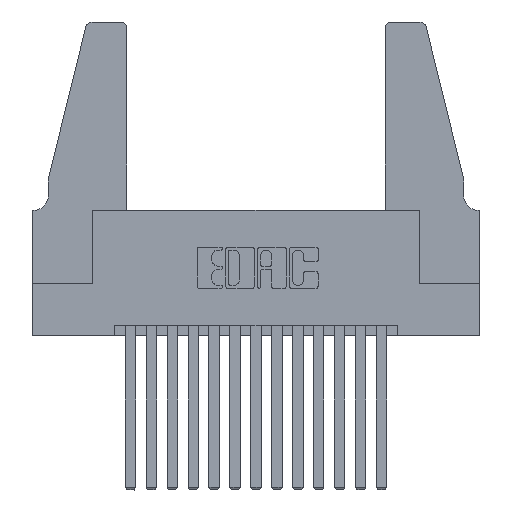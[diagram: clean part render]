
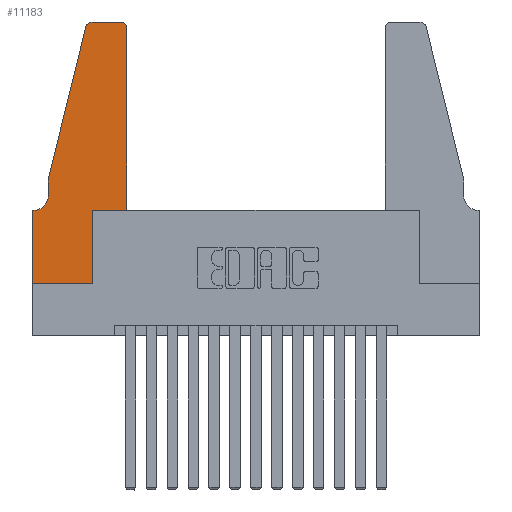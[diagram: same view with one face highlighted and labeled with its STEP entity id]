
A CAD part, top view. The second image highlights one B-rep face of the part: STEP entity #11183.
In plain terms, the highlighted planar face has unit normal (0, 0, 1).
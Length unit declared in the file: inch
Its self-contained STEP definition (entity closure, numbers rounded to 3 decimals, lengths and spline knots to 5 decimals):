
#358 = VERTEX_POINT ( 'NONE', #2515 ) ;
#392 = CARTESIAN_POINT ( 'NONE',  ( 0.0755, 0.42, 0.37 ) ) ;
#960 = VECTOR ( 'NONE', #9195, 39.37008 ) ;
#1009 = LINE ( 'NONE', #8929, #1597 ) ;
#1182 = EDGE_CURVE ( 'NONE', #4025, #11292, #1009, .T. ) ;
#1275 = CARTESIAN_POINT ( 'NONE',  ( 0.4205, 1.25, 0.37 ) ) ;
#1410 = DIRECTION ( 'NONE',  ( 0., 1., 0. ) ) ;
#1597 = VECTOR ( 'NONE', #1410, 39.37008 ) ;
#1605 = EDGE_CURVE ( 'NONE', #15141, #358, #2956, .T. ) ;
#1641 = CARTESIAN_POINT ( 'NONE',  ( 0.0755, 0.5, 0.37 ) ) ;
#1678 = EDGE_CURVE ( 'NONE', #11292, #15141, #5659, .T. ) ;
#1901 = EDGE_CURVE ( 'NONE', #5327, #5474, #14584, .T. ) ;
#1961 = CARTESIAN_POINT ( 'NONE',  ( 0.284, 1.25, 0.37 ) ) ;
#2050 = CARTESIAN_POINT ( 'NONE',  ( 0.0055, 0.35, 0.37 ) ) ;
#2114 = CARTESIAN_POINT ( 'NONE',  ( 0., 0.35, 0.37 ) ) ;
#2127 = DIRECTION ( 'NONE',  ( 0., 0., 1. ) ) ;
#2196 = DIRECTION ( 'NONE',  ( 1., 0., 0. ) ) ;
#2219 = DIRECTION ( 'NONE',  ( -1., 0., 0. ) ) ;
#2321 = CIRCLE ( 'NONE', #5159, 0.03 ) ;
#2365 = ORIENTED_EDGE ( 'NONE', *, *, #8969, .T. ) ;
#2515 = CARTESIAN_POINT ( 'NONE',  ( 0.4505, 1.22, 0.37 ) ) ;
#2618 = VECTOR ( 'NONE', #10276, 39.37008 ) ;
#2921 = VERTEX_POINT ( 'NONE', #392 ) ;
#2956 = LINE ( 'NONE', #7115, #5082 ) ;
#3250 = DIRECTION ( 'NONE',  ( 1., 0., 0. ) ) ;
#3305 = VECTOR ( 'NONE', #12437, 39.37008 ) ;
#3445 = CARTESIAN_POINT ( 'NONE',  ( 0.284, 1.22, 0.37 ) ) ;
#3494 = LINE ( 'NONE', #6681, #960 ) ;
#3738 = EDGE_CURVE ( 'NONE', #2921, #11665, #15704, .T. ) ;
#3867 = ORIENTED_EDGE ( 'NONE', *, *, #1605, .T. ) ;
#4025 = VERTEX_POINT ( 'NONE', #12197 ) ;
#4062 = VERTEX_POINT ( 'NONE', #15067 ) ;
#4244 = LINE ( 'NONE', #9822, #3305 ) ;
#4293 = DIRECTION ( 'NONE',  ( 1., 0., 0. ) ) ;
#4431 = DIRECTION ( 'NONE',  ( 0., 0., 1. ) ) ;
#4722 = CARTESIAN_POINT ( 'NONE',  ( 0.0055, 0.42, 0.37 ) ) ;
#5082 = VECTOR ( 'NONE', #14641, 39.37008 ) ;
#5159 = AXIS2_PLACEMENT_3D ( 'NONE', #13165, #4431, #3250 ) ;
#5327 = VERTEX_POINT ( 'NONE', #1961 ) ;
#5331 = CARTESIAN_POINT ( 'NONE',  ( 0., 0.35, 0.37 ) ) ;
#5474 = VERTEX_POINT ( 'NONE', #7027 ) ;
#5611 = ORIENTED_EDGE ( 'NONE', *, *, #8250, .T. ) ;
#5659 = LINE ( 'NONE', #8253, #8979 ) ;
#5803 = CARTESIAN_POINT ( 'NONE',  ( 0.2605, 1.25, 0.37 ) ) ;
#5871 = DIRECTION ( 'NONE',  ( -1., 0., 0. ) ) ;
#6115 = LINE ( 'NONE', #13977, #9055 ) ;
#6223 = CARTESIAN_POINT ( 'NONE',  ( 0.4505, 0.35, 0.37 ) ) ;
#6244 = ORIENTED_EDGE ( 'NONE', *, *, #13563, .T. ) ;
#6514 = VECTOR ( 'NONE', #2219, 39.37008 ) ;
#6681 = CARTESIAN_POINT ( 'NONE',  ( 0.0755, 0.35, 0.37 ) ) ;
#7027 = CARTESIAN_POINT ( 'NONE',  ( 0.25487, 1.22718, 0.37 ) ) ;
#7115 = CARTESIAN_POINT ( 'NONE',  ( 0.4505, 0.35, 0.37 ) ) ;
#7268 = DIRECTION ( 'NONE',  ( 0., 0., -1. ) ) ;
#7376 = CARTESIAN_POINT ( 'NONE',  ( 0.2865, 0.35, 0.37 ) ) ;
#7581 = ORIENTED_EDGE ( 'NONE', *, *, #12025, .T. ) ;
#8250 = EDGE_CURVE ( 'NONE', #358, #10834, #2321, .T. ) ;
#8253 = CARTESIAN_POINT ( 'NONE',  ( 0.4505, 0.35, 0.37 ) ) ;
#8408 = ORIENTED_EDGE ( 'NONE', *, *, #1678, .T. ) ;
#8537 = VERTEX_POINT ( 'NONE', #13945 ) ;
#8646 = ORIENTED_EDGE ( 'NONE', *, *, #3738, .T. ) ;
#8929 = CARTESIAN_POINT ( 'NONE',  ( 0.2865, 0.35, 0.37 ) ) ;
#8969 = EDGE_CURVE ( 'NONE', #13540, #4062, #4244, .T. ) ;
#8979 = VECTOR ( 'NONE', #13211, 39.37008 ) ;
#9041 = LINE ( 'NONE', #11492, #2618 ) ;
#9055 = VECTOR ( 'NONE', #11519, 39.37008 ) ;
#9088 = EDGE_LOOP ( 'NONE', ( #10732, #14047, #6244, #7581, #8646, #9287, #2365, #9570, #10057, #8408, #3867, #5611 ) ) ;
#9195 = DIRECTION ( 'NONE',  ( -1., 0., 0. ) ) ;
#9287 = ORIENTED_EDGE ( 'NONE', *, *, #14918, .T. ) ;
#9570 = ORIENTED_EDGE ( 'NONE', *, *, #15917, .T. ) ;
#9822 = CARTESIAN_POINT ( 'NONE',  ( 0., 0., 0.37 ) ) ;
#10057 = ORIENTED_EDGE ( 'NONE', *, *, #1182, .T. ) ;
#10241 = DIRECTION ( 'NONE',  ( -0.239, -0.971, 0. ) ) ;
#10276 = DIRECTION ( 'NONE',  ( 0., -1., 0. ) ) ;
#10601 = LINE ( 'NONE', #5803, #6514 ) ;
#10732 = ORIENTED_EDGE ( 'NONE', *, *, #11851, .T. ) ;
#10834 = VERTEX_POINT ( 'NONE', #1275 ) ;
#11183 = ADVANCED_FACE ( 'NONE', ( #14294 ), #11726, .T. ) ;
#11292 = VERTEX_POINT ( 'NONE', #7376 ) ;
#11492 = CARTESIAN_POINT ( 'NONE',  ( 0.0755, 0.5, 0.37 ) ) ;
#11495 = VECTOR ( 'NONE', #10241, 39.37008 ) ;
#11519 = DIRECTION ( 'NONE',  ( 1., 0., 0. ) ) ;
#11665 = VERTEX_POINT ( 'NONE', #2050 ) ;
#11726 = PLANE ( 'NONE',  #13181 ) ;
#11851 = EDGE_CURVE ( 'NONE', #10834, #5327, #10601, .T. ) ;
#12005 = AXIS2_PLACEMENT_3D ( 'NONE', #3445, #2127, #2196 ) ;
#12025 = EDGE_CURVE ( 'NONE', #8537, #2921, #9041, .T. ) ;
#12197 = CARTESIAN_POINT ( 'NONE',  ( 0.2865, 0., 0.37 ) ) ;
#12437 = DIRECTION ( 'NONE',  ( 0., -1., 0. ) ) ;
#13049 = LINE ( 'NONE', #1641, #11495 ) ;
#13165 = CARTESIAN_POINT ( 'NONE',  ( 0.4205, 1.22, 0.37 ) ) ;
#13181 = AXIS2_PLACEMENT_3D ( 'NONE', #2114, #15761, #4293 ) ;
#13211 = DIRECTION ( 'NONE',  ( 1., 0., 0. ) ) ;
#13540 = VERTEX_POINT ( 'NONE', #5331 ) ;
#13563 = EDGE_CURVE ( 'NONE', #5474, #8537, #13049, .T. ) ;
#13945 = CARTESIAN_POINT ( 'NONE',  ( 0.0755, 0.5, 0.37 ) ) ;
#13977 = CARTESIAN_POINT ( 'NONE',  ( 0., 0., 0.37 ) ) ;
#14047 = ORIENTED_EDGE ( 'NONE', *, *, #1901, .T. ) ;
#14294 = FACE_OUTER_BOUND ( 'NONE', #9088, .T. ) ;
#14584 = CIRCLE ( 'NONE', #12005, 0.03 ) ;
#14641 = DIRECTION ( 'NONE',  ( 0., 1., 0. ) ) ;
#14918 = EDGE_CURVE ( 'NONE', #11665, #13540, #3494, .T. ) ;
#15067 = CARTESIAN_POINT ( 'NONE',  ( 0., 0., 0.37 ) ) ;
#15141 = VERTEX_POINT ( 'NONE', #6223 ) ;
#15492 = AXIS2_PLACEMENT_3D ( 'NONE', #4722, #7268, #5871 ) ;
#15704 = CIRCLE ( 'NONE', #15492, 0.07 ) ;
#15761 = DIRECTION ( 'NONE',  ( 0., 0., 1. ) ) ;
#15917 = EDGE_CURVE ( 'NONE', #4062, #4025, #6115, .T. ) ;
